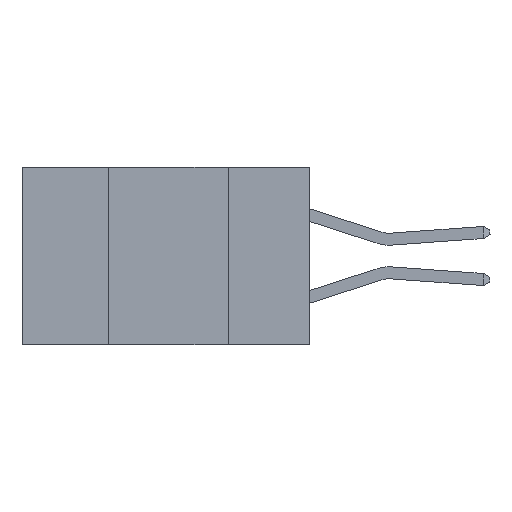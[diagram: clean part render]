
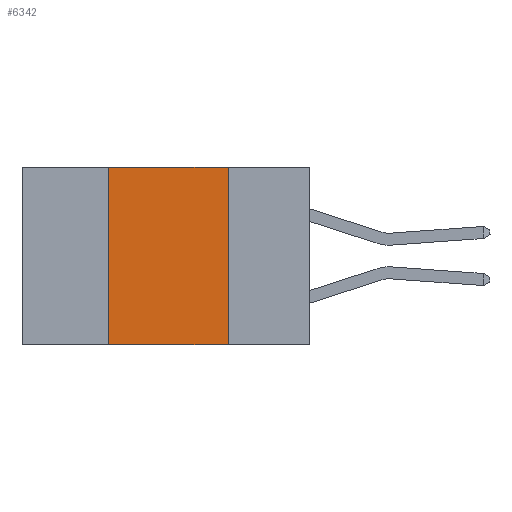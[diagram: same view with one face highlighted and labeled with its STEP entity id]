
A CAD part, left-side view. The second image highlights one B-rep face of the part: STEP entity #6342.
In plain terms, the highlighted planar face has unit normal (-1, 0, 0).
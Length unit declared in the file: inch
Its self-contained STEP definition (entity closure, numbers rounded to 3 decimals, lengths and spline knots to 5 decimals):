
#277 = ORIENTED_EDGE ( 'NONE', *, *, #2998, .F. ) ;
#341 = DIRECTION ( 'NONE',  ( 1., 0., 0. ) ) ;
#604 = VERTEX_POINT ( 'NONE', #11616 ) ;
#1469 = VERTEX_POINT ( 'NONE', #13680 ) ;
#1941 = DIRECTION ( 'NONE',  ( 0., -1., 0. ) ) ;
#2877 = PLANE ( 'NONE',  #27627 ) ;
#2998 = EDGE_CURVE ( 'NONE', #25318, #3824, #7626, .T. ) ;
#3444 = EDGE_CURVE ( 'NONE', #1469, #604, #7596, .T. ) ;
#3824 = VERTEX_POINT ( 'NONE', #28036 ) ;
#5643 = EDGE_CURVE ( 'NONE', #25318, #604, #21159, .T. ) ;
#6342 = ADVANCED_FACE ( 'NONE', ( #32801 ), #2877, .F. ) ;
#7173 = ORIENTED_EDGE ( 'NONE', *, *, #5643, .T. ) ;
#7596 = LINE ( 'NONE', #30803, #13618 ) ;
#7626 = LINE ( 'NONE', #14263, #20555 ) ;
#8880 = VECTOR ( 'NONE', #30633, 39.37008 ) ;
#11616 = CARTESIAN_POINT ( 'NONE',  ( 0., 0.17, -0.37 ) ) ;
#12854 = CARTESIAN_POINT ( 'NONE',  ( 0., 0.6, -0.37 ) ) ;
#13618 = VECTOR ( 'NONE', #20253, 39.37008 ) ;
#13680 = CARTESIAN_POINT ( 'NONE',  ( 0., 0.17, 0. ) ) ;
#13847 = EDGE_LOOP ( 'NONE', ( #23770, #30634, #277, #7173 ) ) ;
#14263 = CARTESIAN_POINT ( 'NONE',  ( 0., 0.42, 0. ) ) ;
#15146 = CARTESIAN_POINT ( 'NONE',  ( 0., 0.6, 0. ) ) ;
#15704 = DIRECTION ( 'NONE',  ( 0., 0., 1. ) ) ;
#16962 = DIRECTION ( 'NONE',  ( 0., 0., -1. ) ) ;
#20253 = DIRECTION ( 'NONE',  ( 0., 0., -1. ) ) ;
#20355 = VECTOR ( 'NONE', #1941, 39.37008 ) ;
#20555 = VECTOR ( 'NONE', #15704, 39.37008 ) ;
#21159 = LINE ( 'NONE', #12854, #20355 ) ;
#21957 = EDGE_CURVE ( 'NONE', #3824, #1469, #28690, .T. ) ;
#23770 = ORIENTED_EDGE ( 'NONE', *, *, #3444, .F. ) ;
#25318 = VERTEX_POINT ( 'NONE', #31398 ) ;
#27627 = AXIS2_PLACEMENT_3D ( 'NONE', #30104, #341, #16962 ) ;
#28036 = CARTESIAN_POINT ( 'NONE',  ( 0., 0.42, 0. ) ) ;
#28690 = LINE ( 'NONE', #15146, #8880 ) ;
#30104 = CARTESIAN_POINT ( 'NONE',  ( 0., 0.6, 0. ) ) ;
#30633 = DIRECTION ( 'NONE',  ( 0., -1., 0. ) ) ;
#30634 = ORIENTED_EDGE ( 'NONE', *, *, #21957, .F. ) ;
#30803 = CARTESIAN_POINT ( 'NONE',  ( 0., 0.17, 0. ) ) ;
#31398 = CARTESIAN_POINT ( 'NONE',  ( 0., 0.42, -0.37 ) ) ;
#32801 = FACE_OUTER_BOUND ( 'NONE', #13847, .T. ) ;
